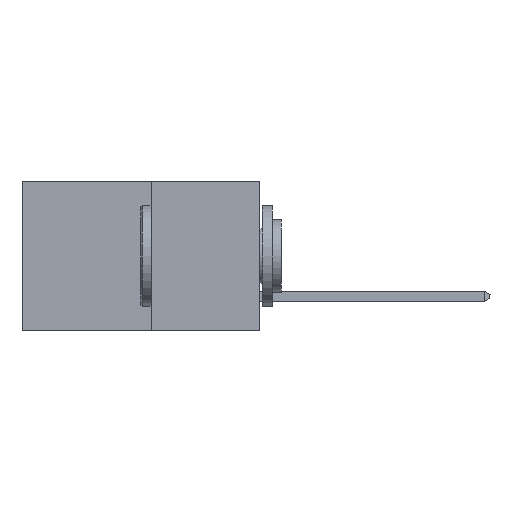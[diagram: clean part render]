
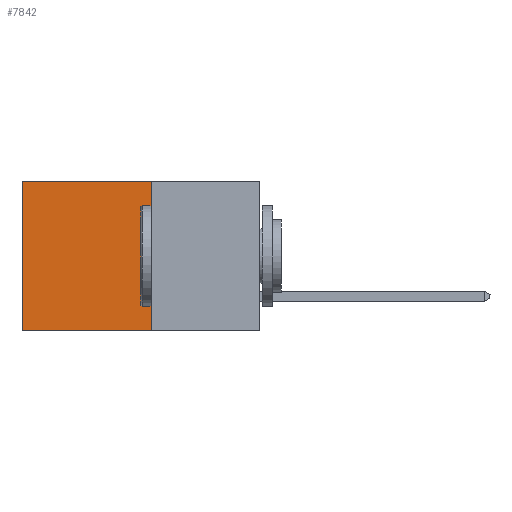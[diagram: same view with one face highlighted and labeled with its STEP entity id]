
A CAD part, left-side view. The second image highlights one B-rep face of the part: STEP entity #7842.
In plain terms, the highlighted planar face has unit normal (-1, 0, 0).
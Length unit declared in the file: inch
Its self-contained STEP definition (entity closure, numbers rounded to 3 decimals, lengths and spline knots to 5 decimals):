
#1590 = ORIENTED_EDGE ( 'NONE', *, *, #3857, .F. ) ;
#1921 = VECTOR ( 'NONE', #11406, 39.37008 ) ;
#2590 = CARTESIAN_POINT ( 'NONE',  ( 0.277, 0.59, 0. ) ) ;
#2743 = EDGE_CURVE ( 'NONE', #3061, #11317, #7558, .T. ) ;
#2794 = EDGE_CURVE ( 'NONE', #5450, #11317, #4457, .T. ) ;
#3061 = VERTEX_POINT ( 'NONE', #9413 ) ;
#3259 = VERTEX_POINT ( 'NONE', #9541 ) ;
#3810 = ORIENTED_EDGE ( 'NONE', *, *, #2794, .T. ) ;
#3857 = EDGE_CURVE ( 'NONE', #3259, #3061, #9555, .T. ) ;
#3964 = CARTESIAN_POINT ( 'NONE',  ( 0.277, 0.59, -0.37 ) ) ;
#4457 = LINE ( 'NONE', #3964, #1921 ) ;
#4591 = DIRECTION ( 'NONE',  ( 0., 0., -1. ) ) ;
#4666 = DIRECTION ( 'NONE',  ( 1., 0., 0. ) ) ;
#4736 = CARTESIAN_POINT ( 'NONE',  ( 0.277, 0.27, -0.37 ) ) ;
#4753 = AXIS2_PLACEMENT_3D ( 'NONE', #4736, #4666, #4591 ) ;
#4858 = PLANE ( 'NONE',  #4753 ) ;
#5450 = VERTEX_POINT ( 'NONE', #2590 ) ;
#5495 = LINE ( 'NONE', #8186, #10159 ) ;
#6473 = EDGE_CURVE ( 'NONE', #3259, #5450, #5495, .T. ) ;
#7078 = FACE_OUTER_BOUND ( 'NONE', #10279, .T. ) ;
#7558 = LINE ( 'NONE', #10105, #12111 ) ;
#7842 = ADVANCED_FACE ( 'NONE', ( #7078 ), #4858, .F. ) ;
#7950 = DIRECTION ( 'NONE',  ( 0., 1., 0. ) ) ;
#8186 = CARTESIAN_POINT ( 'NONE',  ( 0.277, 0.27, 0. ) ) ;
#8850 = ORIENTED_EDGE ( 'NONE', *, *, #2743, .F. ) ;
#9413 = CARTESIAN_POINT ( 'NONE',  ( 0.277, 0.27, -0.37 ) ) ;
#9541 = CARTESIAN_POINT ( 'NONE',  ( 0.277, 0.27, 0. ) ) ;
#9555 = LINE ( 'NONE', #11929, #11664 ) ;
#9846 = DIRECTION ( 'NONE',  ( 0., 1., 0. ) ) ;
#10105 = CARTESIAN_POINT ( 'NONE',  ( 0.277, 0.27, -0.37 ) ) ;
#10159 = VECTOR ( 'NONE', #7950, 39.37008 ) ;
#10279 = EDGE_LOOP ( 'NONE', ( #3810, #8850, #1590, #11521 ) ) ;
#11317 = VERTEX_POINT ( 'NONE', #11876 ) ;
#11406 = DIRECTION ( 'NONE',  ( 0., 0., -1. ) ) ;
#11521 = ORIENTED_EDGE ( 'NONE', *, *, #6473, .T. ) ;
#11664 = VECTOR ( 'NONE', #11958, 39.37008 ) ;
#11876 = CARTESIAN_POINT ( 'NONE',  ( 0.277, 0.59, -0.37 ) ) ;
#11929 = CARTESIAN_POINT ( 'NONE',  ( 0.277, 0.27, -0.37 ) ) ;
#11958 = DIRECTION ( 'NONE',  ( 0., 0., -1. ) ) ;
#12111 = VECTOR ( 'NONE', #9846, 39.37008 ) ;
